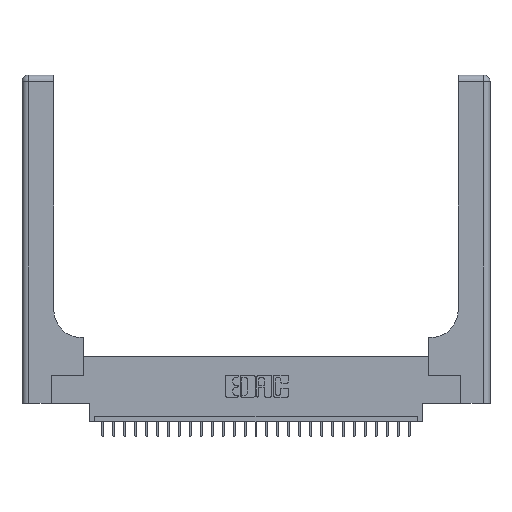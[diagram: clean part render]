
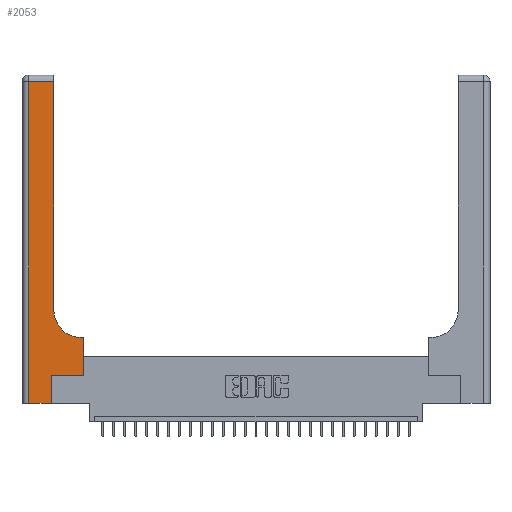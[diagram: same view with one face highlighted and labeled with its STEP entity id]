
A CAD part, top view. The second image highlights one B-rep face of the part: STEP entity #2053.
In plain terms, the highlighted planar face has unit normal (0, 0, 1).
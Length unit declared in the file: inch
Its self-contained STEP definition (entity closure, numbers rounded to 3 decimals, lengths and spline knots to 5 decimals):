
#1206 = DIRECTION ( 'NONE',  ( -1., 0., 0. ) ) ;
#1234 = DIRECTION ( 'NONE',  ( -1., 0., 0. ) ) ;
#1540 = CARTESIAN_POINT ( 'NONE',  ( 0., 2.94, 0.37 ) ) ;
#2053 = ADVANCED_FACE ( 'NONE', ( #17409 ), #10506, .F. ) ;
#2387 = DIRECTION ( 'NONE',  ( 0., 0., -1. ) ) ;
#2659 = DIRECTION ( 'NONE',  ( 1., 0., 0. ) ) ;
#2810 = LINE ( 'NONE', #9839, #4712 ) ;
#2966 = LINE ( 'NONE', #25270, #8844 ) ;
#3423 = LINE ( 'NONE', #17037, #10972 ) ;
#3576 = CARTESIAN_POINT ( 'NONE',  ( 0.2915, 3., 0.37 ) ) ;
#3687 = CARTESIAN_POINT ( 'NONE',  ( 0.5415, 0.6, 0.37 ) ) ;
#3805 = EDGE_CURVE ( 'NONE', #17352, #15577, #12964, .T. ) ;
#4041 = CARTESIAN_POINT ( 'NONE',  ( 0.269, 0.25, 0.37 ) ) ;
#4712 = VECTOR ( 'NONE', #2659, 39.37008 ) ;
#5223 = CARTESIAN_POINT ( 'NONE',  ( 0.269, 0.25, 0.37 ) ) ;
#5262 = EDGE_CURVE ( 'NONE', #26587, #22823, #3423, .T. ) ;
#5532 = CARTESIAN_POINT ( 'NONE',  ( 0.06, 0., 0.37 ) ) ;
#5533 = VECTOR ( 'NONE', #25596, 39.37008 ) ;
#6315 = VERTEX_POINT ( 'NONE', #5532 ) ;
#6637 = ORIENTED_EDGE ( 'NONE', *, *, #11892, .T. ) ;
#6979 = CARTESIAN_POINT ( 'NONE',  ( 0.2915, 0.85, 0.37 ) ) ;
#7176 = ORIENTED_EDGE ( 'NONE', *, *, #9232, .T. ) ;
#8327 = AXIS2_PLACEMENT_3D ( 'NONE', #15562, #2387, #22051 ) ;
#8844 = VECTOR ( 'NONE', #11755, 39.37008 ) ;
#9000 = VERTEX_POINT ( 'NONE', #6979 ) ;
#9126 = EDGE_CURVE ( 'NONE', #19084, #26587, #27495, .T. ) ;
#9232 = EDGE_CURVE ( 'NONE', #17632, #19084, #25454, .T. ) ;
#9673 = ORIENTED_EDGE ( 'NONE', *, *, #5262, .T. ) ;
#9719 = CARTESIAN_POINT ( 'NONE',  ( 0.5585, 0.6, 0.37 ) ) ;
#9839 = CARTESIAN_POINT ( 'NONE',  ( 0., 0., 0.37 ) ) ;
#10143 = ORIENTED_EDGE ( 'NONE', *, *, #27140, .T. ) ;
#10506 = PLANE ( 'NONE',  #15597 ) ;
#10674 = VECTOR ( 'NONE', #14144, 39.37008 ) ;
#10892 = VECTOR ( 'NONE', #19662, 39.37008 ) ;
#10972 = VECTOR ( 'NONE', #1206, 39.37008 ) ;
#11280 = VECTOR ( 'NONE', #21483, 39.37008 ) ;
#11755 = DIRECTION ( 'NONE',  ( 0., 1., 0. ) ) ;
#11892 = EDGE_CURVE ( 'NONE', #17757, #17632, #2966, .T. ) ;
#12356 = VECTOR ( 'NONE', #1234, 39.37008 ) ;
#12964 = LINE ( 'NONE', #1540, #12356 ) ;
#13607 = EDGE_CURVE ( 'NONE', #6315, #17757, #2810, .T. ) ;
#14144 = DIRECTION ( 'NONE',  ( 1., 0., 0. ) ) ;
#14150 = CARTESIAN_POINT ( 'NONE',  ( 0.2915, 2.94, 0.37 ) ) ;
#15562 = CARTESIAN_POINT ( 'NONE',  ( 0.5415, 0.85, 0.37 ) ) ;
#15577 = VERTEX_POINT ( 'NONE', #24163 ) ;
#15597 = AXIS2_PLACEMENT_3D ( 'NONE', #26344, #23869, #26200 ) ;
#16634 = ORIENTED_EDGE ( 'NONE', *, *, #9126, .T. ) ;
#16825 = ORIENTED_EDGE ( 'NONE', *, *, #13607, .T. ) ;
#17037 = CARTESIAN_POINT ( 'NONE',  ( 0.2915, 0.6, 0.37 ) ) ;
#17046 = LINE ( 'NONE', #3576, #11280 ) ;
#17352 = VERTEX_POINT ( 'NONE', #14150 ) ;
#17409 = FACE_OUTER_BOUND ( 'NONE', #25544, .T. ) ;
#17632 = VERTEX_POINT ( 'NONE', #4041 ) ;
#17757 = VERTEX_POINT ( 'NONE', #20459 ) ;
#18108 = EDGE_CURVE ( 'NONE', #22823, #9000, #20995, .T. ) ;
#19084 = VERTEX_POINT ( 'NONE', #25987 ) ;
#19662 = DIRECTION ( 'NONE',  ( 0., -1., 0. ) ) ;
#19801 = LINE ( 'NONE', #26236, #10892 ) ;
#20459 = CARTESIAN_POINT ( 'NONE',  ( 0.269, 0., 0.37 ) ) ;
#20995 = CIRCLE ( 'NONE', #8327, 0.25 ) ;
#21483 = DIRECTION ( 'NONE',  ( 0., 1., 0. ) ) ;
#22051 = DIRECTION ( 'NONE',  ( 1., 0., 0. ) ) ;
#22743 = ORIENTED_EDGE ( 'NONE', *, *, #18108, .T. ) ;
#22823 = VERTEX_POINT ( 'NONE', #3687 ) ;
#23120 = CARTESIAN_POINT ( 'NONE',  ( 0.5585, 0.25, 0.37 ) ) ;
#23572 = EDGE_CURVE ( 'NONE', #9000, #17352, #17046, .T. ) ;
#23869 = DIRECTION ( 'NONE',  ( 0., 0., -1. ) ) ;
#24163 = CARTESIAN_POINT ( 'NONE',  ( 0.06, 2.94, 0.37 ) ) ;
#24730 = ORIENTED_EDGE ( 'NONE', *, *, #23572, .T. ) ;
#25270 = CARTESIAN_POINT ( 'NONE',  ( 0.269, 0., 0.37 ) ) ;
#25454 = LINE ( 'NONE', #5223, #10674 ) ;
#25544 = EDGE_LOOP ( 'NONE', ( #24730, #26729, #10143, #16825, #6637, #7176, #16634, #9673, #22743 ) ) ;
#25596 = DIRECTION ( 'NONE',  ( 0., 1., 0. ) ) ;
#25987 = CARTESIAN_POINT ( 'NONE',  ( 0.5585, 0.25, 0.37 ) ) ;
#26200 = DIRECTION ( 'NONE',  ( -1., 0., 0. ) ) ;
#26236 = CARTESIAN_POINT ( 'NONE',  ( 0.06, 3., 0.37 ) ) ;
#26344 = CARTESIAN_POINT ( 'NONE',  ( 0., 3., 0.37 ) ) ;
#26587 = VERTEX_POINT ( 'NONE', #9719 ) ;
#26729 = ORIENTED_EDGE ( 'NONE', *, *, #3805, .T. ) ;
#27140 = EDGE_CURVE ( 'NONE', #15577, #6315, #19801, .T. ) ;
#27495 = LINE ( 'NONE', #23120, #5533 ) ;
